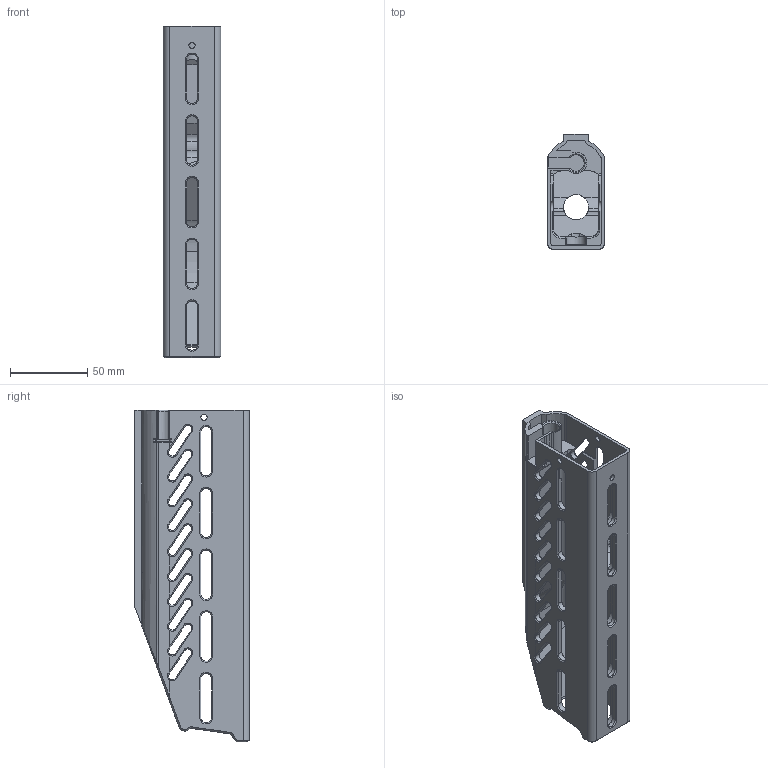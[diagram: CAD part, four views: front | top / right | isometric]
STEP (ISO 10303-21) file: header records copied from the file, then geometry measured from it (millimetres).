
FILE_DESCRIPTION(/* description */ (''),/* implementation_level */ '2;1');
FILE_NAME(/* name */ 'Hand Guard.step',/* time_stamp */ '2022-05-11T21:20:06-06:00',/* author */ (''),/* organization */ (''),/* preprocessor_version */ 'ST-DEVELOPER v18.1',/* originating_system */ 'Autodesk Translation Framework v10.10.0.1391',/* authorisation */ '');
FILE_SCHEMA (('AUTOMOTIVE_DESIGN { 1 0 10303 214 3 1 1 }'));
Length unit declared in the file: millimetre
Products named in the file (1): Vented Handguard.
Bounding box: 37.08 x 74.44 x 215 mm (x, y, z)
Volume: 178705.9 mm3; surface area: 81837.5 mm2
Topology: 1 solids, 1 shells, 608 faces, 1765 edges, 1126 vertices
Faces by surface type: plane 313, cylinder 148, cone 77, bspline 66, torus 4
Full cylindrical faces by diameter (mm): 3 x4, 4 x3, 4.5 x3, 4.748 x1, 5 x1, 16.3 x1
Entity records: 21820 total; most frequent: CARTESIAN_POINT 5924, ORIENTED_EDGE 3530, DIRECTION 3047, EDGE_CURVE 1765, LINE 1141, VECTOR 1141, VERTEX_POINT 1126, AXIS2_PLACEMENT_3D 953
